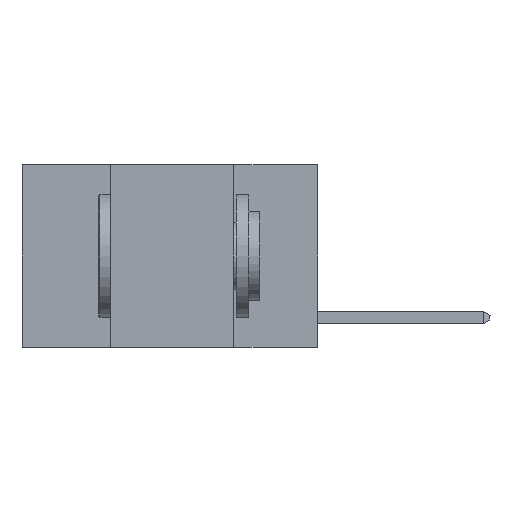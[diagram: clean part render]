
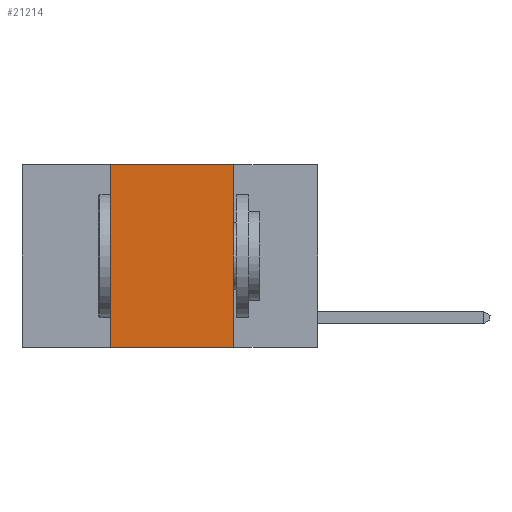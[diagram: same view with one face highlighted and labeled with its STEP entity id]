
A CAD part, left-side view. The second image highlights one B-rep face of the part: STEP entity #21214.
In plain terms, the highlighted planar face has unit normal (-1, 0, 0).
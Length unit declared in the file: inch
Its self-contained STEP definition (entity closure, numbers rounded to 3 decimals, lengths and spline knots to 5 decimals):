
#373 = EDGE_CURVE ( 'NONE', #11868, #1409, #1637, .T. ) ;
#1040 = DIRECTION ( 'NONE',  ( 1., 0., 0. ) ) ;
#1239 = DIRECTION ( 'NONE',  ( 0., 0., -1. ) ) ;
#1302 = EDGE_CURVE ( 'NONE', #2317, #19505, #18279, .T. ) ;
#1409 = VERTEX_POINT ( 'NONE', #9047 ) ;
#1517 = DIRECTION ( 'NONE',  ( 0., 0., -1. ) ) ;
#1637 = LINE ( 'NONE', #8369, #4558 ) ;
#1910 = VECTOR ( 'NONE', #3522, 39.37008 ) ;
#2211 = CARTESIAN_POINT ( 'NONE',  ( 0., 0.6, -0.37 ) ) ;
#2317 = VERTEX_POINT ( 'NONE', #17011 ) ;
#3278 = CARTESIAN_POINT ( 'NONE',  ( 0., 0.42, 0. ) ) ;
#3522 = DIRECTION ( 'NONE',  ( 0., -1., 0. ) ) ;
#3611 = EDGE_CURVE ( 'NONE', #2317, #1409, #12213, .T. ) ;
#3924 = VECTOR ( 'NONE', #9916, 39.37008 ) ;
#4558 = VECTOR ( 'NONE', #1517, 39.37008 ) ;
#5712 = CARTESIAN_POINT ( 'NONE',  ( 0., 0.6, 0. ) ) ;
#5772 = CARTESIAN_POINT ( 'NONE',  ( 0., 0.17, 0. ) ) ;
#6785 = ORIENTED_EDGE ( 'NONE', *, *, #11445, .F. ) ;
#8369 = CARTESIAN_POINT ( 'NONE',  ( 0., 0.17, 0. ) ) ;
#9047 = CARTESIAN_POINT ( 'NONE',  ( 0., 0.17, -0.37 ) ) ;
#9297 = AXIS2_PLACEMENT_3D ( 'NONE', #9502, #1040, #1239 ) ;
#9502 = CARTESIAN_POINT ( 'NONE',  ( 0., 0.6, 0. ) ) ;
#9916 = DIRECTION ( 'NONE',  ( 0., 0., 1. ) ) ;
#11125 = FACE_OUTER_BOUND ( 'NONE', #15811, .T. ) ;
#11445 = EDGE_CURVE ( 'NONE', #19505, #11868, #20594, .T. ) ;
#11868 = VERTEX_POINT ( 'NONE', #5772 ) ;
#11954 = ORIENTED_EDGE ( 'NONE', *, *, #373, .F. ) ;
#12213 = LINE ( 'NONE', #2211, #1910 ) ;
#12350 = DIRECTION ( 'NONE',  ( 0., -1., 0. ) ) ;
#15811 = EDGE_LOOP ( 'NONE', ( #11954, #6785, #16153, #18283 ) ) ;
#15910 = PLANE ( 'NONE',  #9297 ) ;
#16153 = ORIENTED_EDGE ( 'NONE', *, *, #1302, .F. ) ;
#16760 = VECTOR ( 'NONE', #12350, 39.37008 ) ;
#17011 = CARTESIAN_POINT ( 'NONE',  ( 0., 0.42, -0.37 ) ) ;
#17512 = CARTESIAN_POINT ( 'NONE',  ( 0., 0.42, 0. ) ) ;
#18279 = LINE ( 'NONE', #3278, #3924 ) ;
#18283 = ORIENTED_EDGE ( 'NONE', *, *, #3611, .T. ) ;
#19505 = VERTEX_POINT ( 'NONE', #17512 ) ;
#20594 = LINE ( 'NONE', #5712, #16760 ) ;
#21214 = ADVANCED_FACE ( 'NONE', ( #11125 ), #15910, .F. ) ;
